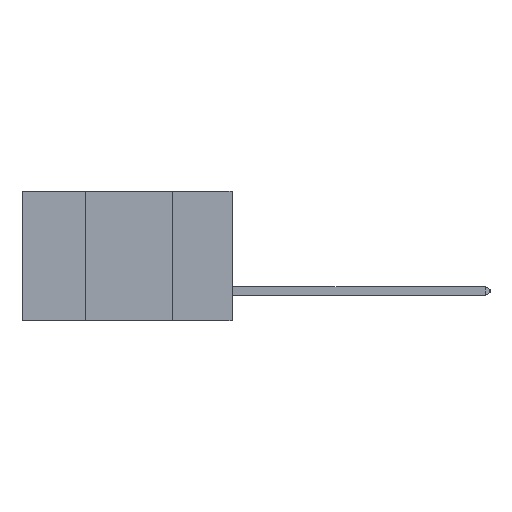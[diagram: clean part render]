
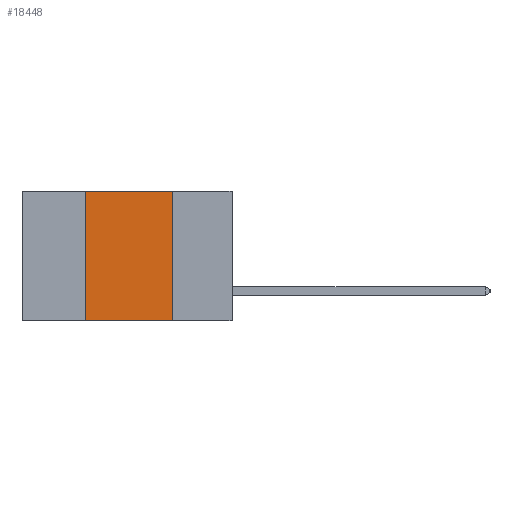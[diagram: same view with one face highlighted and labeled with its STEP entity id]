
A CAD part, left-side view. The second image highlights one B-rep face of the part: STEP entity #18448.
In plain terms, the highlighted planar face has unit normal (-1, 0, 0).
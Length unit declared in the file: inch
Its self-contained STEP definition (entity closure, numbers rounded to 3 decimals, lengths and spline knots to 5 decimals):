
#2009 = EDGE_CURVE ( 'NONE', #15665, #5751, #12186, .T. ) ;
#3336 = EDGE_CURVE ( 'NONE', #15665, #8261, #5702, .T. ) ;
#3802 = CARTESIAN_POINT ( 'NONE',  ( 0., 0.17, -0.37 ) ) ;
#4101 = FACE_OUTER_BOUND ( 'NONE', #4330, .T. ) ;
#4330 = EDGE_LOOP ( 'NONE', ( #13200, #8237, #13416, #21381 ) ) ;
#4619 = EDGE_CURVE ( 'NONE', #14786, #5751, #20111, .T. ) ;
#4736 = VECTOR ( 'NONE', #15765, 39.37008 ) ;
#5371 = CARTESIAN_POINT ( 'NONE',  ( 0., 0.42, 0. ) ) ;
#5702 = LINE ( 'NONE', #5371, #10047 ) ;
#5751 = VERTEX_POINT ( 'NONE', #3802 ) ;
#7063 = DIRECTION ( 'NONE',  ( 1., 0., 0. ) ) ;
#8077 = CARTESIAN_POINT ( 'NONE',  ( 0., 0.42, -0.37 ) ) ;
#8237 = ORIENTED_EDGE ( 'NONE', *, *, #12445, .F. ) ;
#8261 = VERTEX_POINT ( 'NONE', #10812 ) ;
#8280 = LINE ( 'NONE', #20892, #22363 ) ;
#8419 = DIRECTION ( 'NONE',  ( 0., 0., 1. ) ) ;
#8844 = PLANE ( 'NONE',  #16199 ) ;
#8972 = CARTESIAN_POINT ( 'NONE',  ( 0., 0.6, -0.37 ) ) ;
#9666 = DIRECTION ( 'NONE',  ( 0., -1., 0. ) ) ;
#10047 = VECTOR ( 'NONE', #8419, 39.37008 ) ;
#10812 = CARTESIAN_POINT ( 'NONE',  ( 0., 0.42, 0. ) ) ;
#11738 = DIRECTION ( 'NONE',  ( 0., -1., 0. ) ) ;
#12186 = LINE ( 'NONE', #8972, #17123 ) ;
#12445 = EDGE_CURVE ( 'NONE', #8261, #14786, #8280, .T. ) ;
#13200 = ORIENTED_EDGE ( 'NONE', *, *, #4619, .F. ) ;
#13416 = ORIENTED_EDGE ( 'NONE', *, *, #3336, .F. ) ;
#14786 = VERTEX_POINT ( 'NONE', #16481 ) ;
#15665 = VERTEX_POINT ( 'NONE', #8077 ) ;
#15765 = DIRECTION ( 'NONE',  ( 0., 0., -1. ) ) ;
#16199 = AXIS2_PLACEMENT_3D ( 'NONE', #18212, #7063, #19994 ) ;
#16481 = CARTESIAN_POINT ( 'NONE',  ( 0., 0.17, 0. ) ) ;
#17123 = VECTOR ( 'NONE', #9666, 39.37008 ) ;
#18212 = CARTESIAN_POINT ( 'NONE',  ( 0., 0.6, 0. ) ) ;
#18448 = ADVANCED_FACE ( 'NONE', ( #4101 ), #8844, .F. ) ;
#19994 = DIRECTION ( 'NONE',  ( 0., 0., -1. ) ) ;
#20111 = LINE ( 'NONE', #20626, #4736 ) ;
#20626 = CARTESIAN_POINT ( 'NONE',  ( 0., 0.17, 0. ) ) ;
#20892 = CARTESIAN_POINT ( 'NONE',  ( 0., 0.6, 0. ) ) ;
#21381 = ORIENTED_EDGE ( 'NONE', *, *, #2009, .T. ) ;
#22363 = VECTOR ( 'NONE', #11738, 39.37008 ) ;
